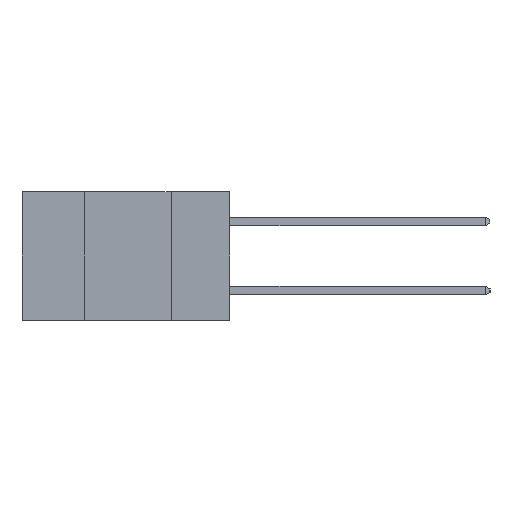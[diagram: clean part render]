
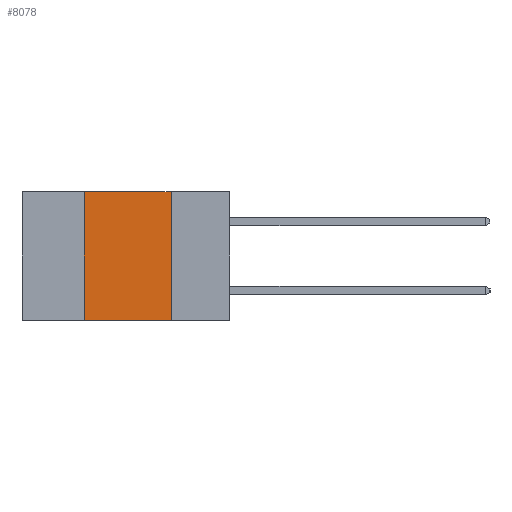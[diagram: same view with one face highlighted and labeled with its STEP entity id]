
A CAD part, left-side view. The second image highlights one B-rep face of the part: STEP entity #8078.
In plain terms, the highlighted planar face has unit normal (-1, 0, 0).
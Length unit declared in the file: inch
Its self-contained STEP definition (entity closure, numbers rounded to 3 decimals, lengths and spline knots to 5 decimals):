
#80 = VERTEX_POINT ( 'NONE', #2625 ) ;
#1445 = ORIENTED_EDGE ( 'NONE', *, *, #9797, .F. ) ;
#2326 = FACE_OUTER_BOUND ( 'NONE', #8798, .T. ) ;
#2359 = DIRECTION ( 'NONE',  ( 0., 0., -1. ) ) ;
#2625 = CARTESIAN_POINT ( 'NONE',  ( 0., 0.17, -0.37 ) ) ;
#2663 = LINE ( 'NONE', #8406, #8362 ) ;
#2767 = DIRECTION ( 'NONE',  ( 0., -1., 0. ) ) ;
#3182 = AXIS2_PLACEMENT_3D ( 'NONE', #4603, #6936, #5389 ) ;
#3190 = EDGE_CURVE ( 'NONE', #5142, #9868, #2663, .T. ) ;
#3699 = EDGE_CURVE ( 'NONE', #5142, #80, #7728, .T. ) ;
#4270 = ORIENTED_EDGE ( 'NONE', *, *, #3699, .T. ) ;
#4603 = CARTESIAN_POINT ( 'NONE',  ( 0., 0.6, 0. ) ) ;
#4606 = VECTOR ( 'NONE', #2359, 39.37008 ) ;
#4716 = PLANE ( 'NONE',  #3182 ) ;
#4834 = DIRECTION ( 'NONE',  ( 0., -1., 0. ) ) ;
#5142 = VERTEX_POINT ( 'NONE', #7084 ) ;
#5389 = DIRECTION ( 'NONE',  ( 0., 0., -1. ) ) ;
#6936 = DIRECTION ( 'NONE',  ( 1., 0., 0. ) ) ;
#7084 = CARTESIAN_POINT ( 'NONE',  ( 0., 0.42, -0.37 ) ) ;
#7266 = EDGE_CURVE ( 'NONE', #9868, #7829, #7795, .T. ) ;
#7331 = ORIENTED_EDGE ( 'NONE', *, *, #7266, .F. ) ;
#7728 = LINE ( 'NONE', #8862, #8352 ) ;
#7795 = LINE ( 'NONE', #7984, #9364 ) ;
#7829 = VERTEX_POINT ( 'NONE', #9341 ) ;
#7889 = LINE ( 'NONE', #9126, #4606 ) ;
#7984 = CARTESIAN_POINT ( 'NONE',  ( 0., 0.6, 0. ) ) ;
#8078 = ADVANCED_FACE ( 'NONE', ( #2326 ), #4716, .F. ) ;
#8352 = VECTOR ( 'NONE', #2767, 39.37008 ) ;
#8362 = VECTOR ( 'NONE', #9898, 39.37008 ) ;
#8406 = CARTESIAN_POINT ( 'NONE',  ( 0., 0.42, -0.37 ) ) ;
#8611 = CARTESIAN_POINT ( 'NONE',  ( 0., 0.42, 0. ) ) ;
#8798 = EDGE_LOOP ( 'NONE', ( #1445, #7331, #9030, #4270 ) ) ;
#8862 = CARTESIAN_POINT ( 'NONE',  ( 0., 0.6, -0.37 ) ) ;
#9030 = ORIENTED_EDGE ( 'NONE', *, *, #3190, .F. ) ;
#9126 = CARTESIAN_POINT ( 'NONE',  ( 0., 0.17, -0.37 ) ) ;
#9341 = CARTESIAN_POINT ( 'NONE',  ( 0., 0.17, 0. ) ) ;
#9364 = VECTOR ( 'NONE', #4834, 39.37008 ) ;
#9797 = EDGE_CURVE ( 'NONE', #7829, #80, #7889, .T. ) ;
#9868 = VERTEX_POINT ( 'NONE', #8611 ) ;
#9898 = DIRECTION ( 'NONE',  ( 0., 0., 1. ) ) ;
